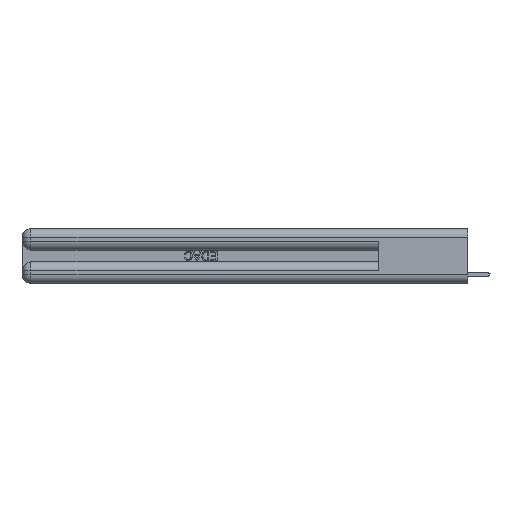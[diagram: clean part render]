
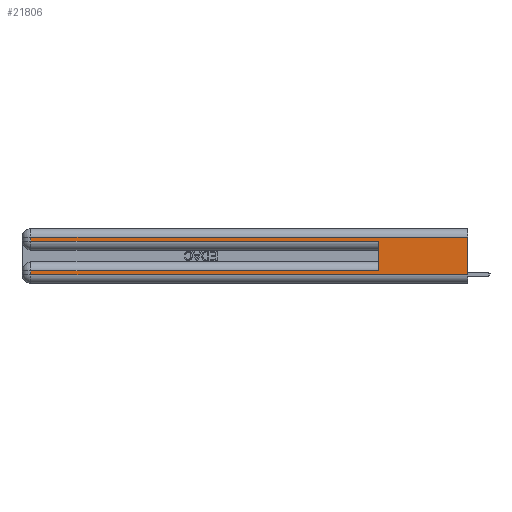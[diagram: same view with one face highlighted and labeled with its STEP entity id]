
A CAD part, left-side view. The second image highlights one B-rep face of the part: STEP entity #21806.
In plain terms, the highlighted planar face has unit normal (-1, 0, 0).
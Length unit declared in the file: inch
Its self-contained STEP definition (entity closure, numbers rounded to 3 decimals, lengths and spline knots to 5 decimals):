
#298 = LINE ( 'NONE', #20039, #7787 ) ;
#617 = DIRECTION ( 'NONE',  ( 0., 0., -1. ) ) ;
#835 = EDGE_CURVE ( 'NONE', #24333, #10912, #11355, .T. ) ;
#1127 = VECTOR ( 'NONE', #4500, 39.37008 ) ;
#1680 = VERTEX_POINT ( 'NONE', #12227 ) ;
#1980 = ORIENTED_EDGE ( 'NONE', *, *, #26085, .T. ) ;
#2838 = EDGE_CURVE ( 'NONE', #6468, #10912, #8967, .T. ) ;
#3043 = PLANE ( 'NONE',  #17845 ) ;
#3101 = VERTEX_POINT ( 'NONE', #11484 ) ;
#3757 = CARTESIAN_POINT ( 'NONE',  ( 0., 2.94, 0.085 ) ) ;
#3961 = EDGE_CURVE ( 'NONE', #28657, #24333, #7447, .T. ) ;
#4500 = DIRECTION ( 'NONE',  ( 0., -1., 0. ) ) ;
#5260 = VECTOR ( 'NONE', #26439, 39.37008 ) ;
#5298 = VECTOR ( 'NONE', #13132, 39.37008 ) ;
#6468 = VERTEX_POINT ( 'NONE', #13334 ) ;
#7447 = LINE ( 'NONE', #10641, #5260 ) ;
#7540 = DIRECTION ( 'NONE',  ( 0., 0., -1. ) ) ;
#7787 = VECTOR ( 'NONE', #19837, 39.37008 ) ;
#8020 = FACE_OUTER_BOUND ( 'NONE', #25863, .T. ) ;
#8400 = ORIENTED_EDGE ( 'NONE', *, *, #28658, .T. ) ;
#8562 = LINE ( 'NONE', #14415, #25819 ) ;
#8842 = VECTOR ( 'NONE', #617, 39.37008 ) ;
#8858 = EDGE_CURVE ( 'NONE', #1680, #20286, #14424, .T. ) ;
#8967 = LINE ( 'NONE', #11052, #28694 ) ;
#9687 = CARTESIAN_POINT ( 'NONE',  ( 0., 0., 0.37 ) ) ;
#9745 = DIRECTION ( 'NONE',  ( 0., 1., 0. ) ) ;
#10641 = CARTESIAN_POINT ( 'NONE',  ( 0., 2.94, 0.37 ) ) ;
#10642 = CARTESIAN_POINT ( 'NONE',  ( 0., 0., 0.285 ) ) ;
#10655 = ORIENTED_EDGE ( 'NONE', *, *, #2838, .F. ) ;
#10912 = VERTEX_POINT ( 'NONE', #25666 ) ;
#11052 = CARTESIAN_POINT ( 'NONE',  ( 0., 0.6, 0.145 ) ) ;
#11355 = LINE ( 'NONE', #10642, #5298 ) ;
#11442 = VERTEX_POINT ( 'NONE', #3757 ) ;
#11484 = CARTESIAN_POINT ( 'NONE',  ( 0., 2.94, 0.06 ) ) ;
#11696 = DIRECTION ( 'NONE',  ( 0., 0., -1. ) ) ;
#12227 = CARTESIAN_POINT ( 'NONE',  ( 0., 0., 0.31 ) ) ;
#13132 = DIRECTION ( 'NONE',  ( 0., -1., 0. ) ) ;
#13334 = CARTESIAN_POINT ( 'NONE',  ( 0., 0.6, 0.085 ) ) ;
#14059 = DIRECTION ( 'NONE',  ( 1., 0., 0. ) ) ;
#14258 = CARTESIAN_POINT ( 'NONE',  ( 0., 0., 0.37 ) ) ;
#14415 = CARTESIAN_POINT ( 'NONE',  ( 0., 0., 0.31 ) ) ;
#14424 = LINE ( 'NONE', #9687, #16877 ) ;
#15692 = DIRECTION ( 'NONE',  ( 0., 0., 1. ) ) ;
#16877 = VECTOR ( 'NONE', #7540, 39.37008 ) ;
#17717 = EDGE_CURVE ( 'NONE', #11442, #3101, #22943, .T. ) ;
#17845 = AXIS2_PLACEMENT_3D ( 'NONE', #14258, #14059, #11696 ) ;
#19621 = CARTESIAN_POINT ( 'NONE',  ( 0., 0., 0.06 ) ) ;
#19837 = DIRECTION ( 'NONE',  ( 0., 1., 0. ) ) ;
#20039 = CARTESIAN_POINT ( 'NONE',  ( 0., 0., 0.085 ) ) ;
#20286 = VERTEX_POINT ( 'NONE', #19621 ) ;
#21806 = ADVANCED_FACE ( 'NONE', ( #8020 ), #3043, .F. ) ;
#22422 = CARTESIAN_POINT ( 'NONE',  ( 0., 0., 0.06 ) ) ;
#22887 = ORIENTED_EDGE ( 'NONE', *, *, #27336, .T. ) ;
#22917 = ORIENTED_EDGE ( 'NONE', *, *, #835, .T. ) ;
#22943 = LINE ( 'NONE', #25345, #8842 ) ;
#23286 = ORIENTED_EDGE ( 'NONE', *, *, #3961, .T. ) ;
#24333 = VERTEX_POINT ( 'NONE', #29334 ) ;
#25345 = CARTESIAN_POINT ( 'NONE',  ( 0., 2.94, 0.37 ) ) ;
#25666 = CARTESIAN_POINT ( 'NONE',  ( 0., 0.6, 0.285 ) ) ;
#25816 = CARTESIAN_POINT ( 'NONE',  ( 0., 2.94, 0.31 ) ) ;
#25819 = VECTOR ( 'NONE', #9745, 39.37008 ) ;
#25863 = EDGE_LOOP ( 'NONE', ( #29079, #8400, #23286, #22917, #10655, #1980, #25998, #22887 ) ) ;
#25998 = ORIENTED_EDGE ( 'NONE', *, *, #17717, .T. ) ;
#26085 = EDGE_CURVE ( 'NONE', #6468, #11442, #298, .T. ) ;
#26439 = DIRECTION ( 'NONE',  ( 0., 0., -1. ) ) ;
#27336 = EDGE_CURVE ( 'NONE', #3101, #20286, #27347, .T. ) ;
#27347 = LINE ( 'NONE', #22422, #1127 ) ;
#28657 = VERTEX_POINT ( 'NONE', #25816 ) ;
#28658 = EDGE_CURVE ( 'NONE', #1680, #28657, #8562, .T. ) ;
#28694 = VECTOR ( 'NONE', #15692, 39.37008 ) ;
#29079 = ORIENTED_EDGE ( 'NONE', *, *, #8858, .F. ) ;
#29334 = CARTESIAN_POINT ( 'NONE',  ( 0., 2.94, 0.285 ) ) ;
